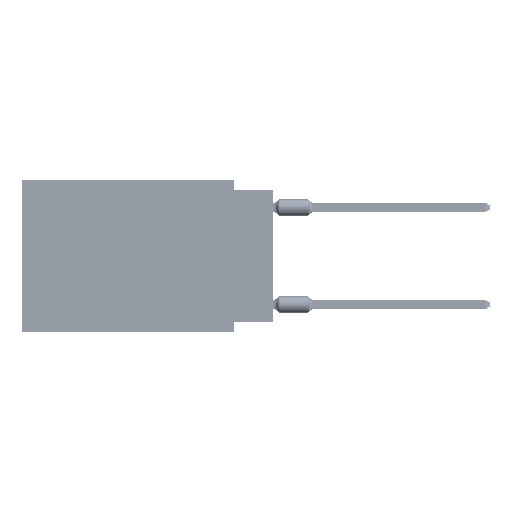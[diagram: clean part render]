
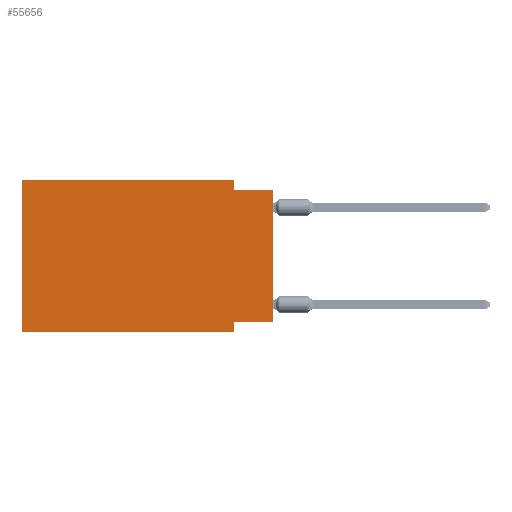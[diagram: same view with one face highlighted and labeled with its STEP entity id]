
A CAD part, left-side view. The second image highlights one B-rep face of the part: STEP entity #55656.
In plain terms, the highlighted planar face has unit normal (-1, 0, 0).
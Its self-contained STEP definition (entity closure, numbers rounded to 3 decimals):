
#449 = EDGE_CURVE ( 'NONE', #42414, #69366, #58956, .T. ) ;
#992 = PLANE ( 'NONE',  #9971 ) ;
#1370 = VERTEX_POINT ( 'NONE', #67418 ) ;
#1612 = DIRECTION ( 'NONE',  ( 0., 0., -1. ) ) ;
#2847 = CARTESIAN_POINT ( 'NONE',  ( 0., 0., -0.635 ) ) ;
#5189 = VECTOR ( 'NONE', #14220, 1000. ) ;
#6039 = EDGE_CURVE ( 'NONE', #20680, #1370, #68649, .T. ) ;
#7061 = LINE ( 'NONE', #18314, #5189 ) ;
#7072 = ORIENTED_EDGE ( 'NONE', *, *, #32611, .F. ) ;
#8313 = DIRECTION ( 'NONE',  ( 0., -1., 0. ) ) ;
#9282 = CARTESIAN_POINT ( 'NONE',  ( 0., 2.54, -9.906 ) ) ;
#9504 = CARTESIAN_POINT ( 'NONE',  ( 0., 0., 0. ) ) ;
#9971 = AXIS2_PLACEMENT_3D ( 'NONE', #68555, #52188, #40936 ) ;
#10782 = EDGE_CURVE ( 'NONE', #57472, #14992, #68110, .T. ) ;
#11078 = VERTEX_POINT ( 'NONE', #37048 ) ;
#11307 = ORIENTED_EDGE ( 'NONE', *, *, #449, .T. ) ;
#11381 = LINE ( 'NONE', #66255, #44944 ) ;
#11429 = VECTOR ( 'NONE', #70185, 1000. ) ;
#14083 = ORIENTED_EDGE ( 'NONE', *, *, #59339, .T. ) ;
#14220 = DIRECTION ( 'NONE',  ( 0., -1., 0. ) ) ;
#14992 = VERTEX_POINT ( 'NONE', #47199 ) ;
#16592 = EDGE_CURVE ( 'NONE', #11078, #57472, #7061, .T. ) ;
#18314 = CARTESIAN_POINT ( 'NONE',  ( 0., 16.383, 0. ) ) ;
#20680 = VERTEX_POINT ( 'NONE', #52163 ) ;
#21990 = EDGE_LOOP ( 'NONE', ( #14083, #7072, #54460, #62070, #55384, #11307, #35102, #22715 ) ) ;
#22715 = ORIENTED_EDGE ( 'NONE', *, *, #6039, .F. ) ;
#24893 = CARTESIAN_POINT ( 'NONE',  ( 0., 0., -0.635 ) ) ;
#26694 = VECTOR ( 'NONE', #66250, 1000. ) ;
#27361 = VERTEX_POINT ( 'NONE', #24893 ) ;
#29225 = CARTESIAN_POINT ( 'NONE',  ( 0., 2.54, 0. ) ) ;
#30238 = DIRECTION ( 'NONE',  ( 0., -1., 0. ) ) ;
#32611 = EDGE_CURVE ( 'NONE', #14992, #27361, #52635, .T. ) ;
#35102 = ORIENTED_EDGE ( 'NONE', *, *, #36684, .F. ) ;
#35241 = CARTESIAN_POINT ( 'NONE',  ( 0., 0., -9.271 ) ) ;
#36684 = EDGE_CURVE ( 'NONE', #1370, #69366, #47791, .T. ) ;
#37048 = CARTESIAN_POINT ( 'NONE',  ( 0., 16.383, 0. ) ) ;
#40451 = VECTOR ( 'NONE', #8313, 1000. ) ;
#40936 = DIRECTION ( 'NONE',  ( 0., 0., -1. ) ) ;
#42414 = VERTEX_POINT ( 'NONE', #70078 ) ;
#44944 = VECTOR ( 'NONE', #60068, 1000. ) ;
#47199 = CARTESIAN_POINT ( 'NONE',  ( 0., 2.54, -0.635 ) ) ;
#47744 = CARTESIAN_POINT ( 'NONE',  ( 0., 2.54, 0. ) ) ;
#47791 = LINE ( 'NONE', #9282, #68727 ) ;
#48009 = CARTESIAN_POINT ( 'NONE',  ( 0., 2.54, -9.906 ) ) ;
#48017 = LINE ( 'NONE', #9504, #11429 ) ;
#49468 = VECTOR ( 'NONE', #30238, 1000. ) ;
#51475 = FACE_OUTER_BOUND ( 'NONE', #21990, .T. ) ;
#52163 = CARTESIAN_POINT ( 'NONE',  ( 0., 0., -9.271 ) ) ;
#52188 = DIRECTION ( 'NONE',  ( 1., 0., 0. ) ) ;
#52635 = LINE ( 'NONE', #2847, #40451 ) ;
#53139 = CARTESIAN_POINT ( 'NONE',  ( 0., 16.383, -9.906 ) ) ;
#54460 = ORIENTED_EDGE ( 'NONE', *, *, #10782, .F. ) ;
#55384 = ORIENTED_EDGE ( 'NONE', *, *, #57526, .F. ) ;
#55656 = ADVANCED_FACE ( 'NONE', ( #51475 ), #992, .F. ) ;
#57472 = VERTEX_POINT ( 'NONE', #47744 ) ;
#57526 = EDGE_CURVE ( 'NONE', #42414, #11078, #11381, .T. ) ;
#58956 = LINE ( 'NONE', #53139, #49468 ) ;
#59339 = EDGE_CURVE ( 'NONE', #20680, #27361, #48017, .T. ) ;
#60068 = DIRECTION ( 'NONE',  ( 0., 0., 1. ) ) ;
#61940 = VECTOR ( 'NONE', #1612, 1000. ) ;
#62070 = ORIENTED_EDGE ( 'NONE', *, *, #16592, .F. ) ;
#66250 = DIRECTION ( 'NONE',  ( 0., 1., 0. ) ) ;
#66255 = CARTESIAN_POINT ( 'NONE',  ( 0., 16.383, 0. ) ) ;
#67418 = CARTESIAN_POINT ( 'NONE',  ( 0., 2.54, -9.271 ) ) ;
#68110 = LINE ( 'NONE', #29225, #61940 ) ;
#68555 = CARTESIAN_POINT ( 'NONE',  ( 0., 16.383, 0. ) ) ;
#68649 = LINE ( 'NONE', #35241, #26694 ) ;
#68727 = VECTOR ( 'NONE', #71387, 1000. ) ;
#69366 = VERTEX_POINT ( 'NONE', #48009 ) ;
#70078 = CARTESIAN_POINT ( 'NONE',  ( 0., 16.383, -9.906 ) ) ;
#70185 = DIRECTION ( 'NONE',  ( 0., 0., 1. ) ) ;
#71387 = DIRECTION ( 'NONE',  ( 0., 0., -1. ) ) ;
